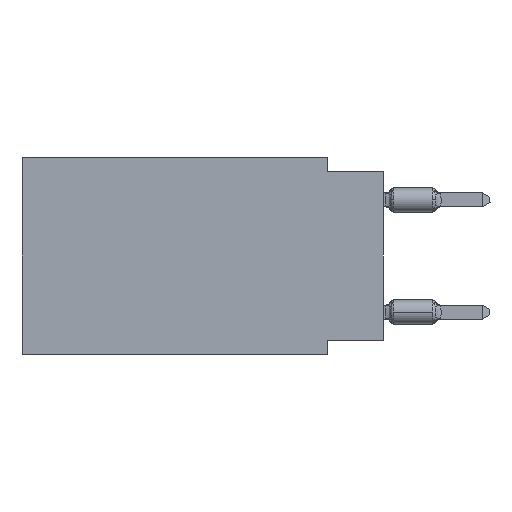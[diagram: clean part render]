
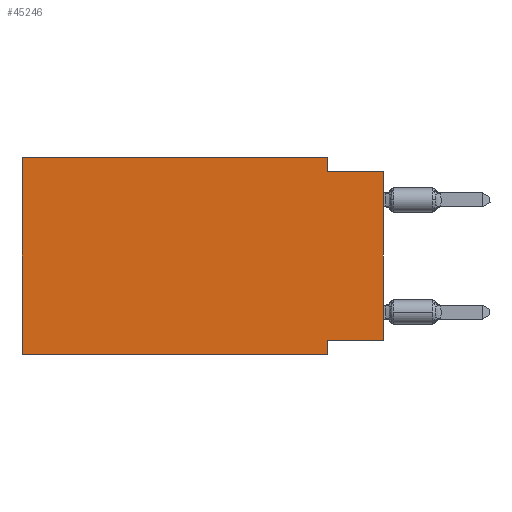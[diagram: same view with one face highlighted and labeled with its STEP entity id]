
A CAD part, left-side view. The second image highlights one B-rep face of the part: STEP entity #45246.
In plain terms, the highlighted planar face has unit normal (-1, 0, 0).
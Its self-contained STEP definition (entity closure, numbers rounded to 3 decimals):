
#296 = EDGE_CURVE ( 'NONE', #33533, #3834, #25748, .T. ) ;
#450 = EDGE_CURVE ( 'NONE', #44304, #37384, #37799, .T. ) ;
#737 = EDGE_CURVE ( 'NONE', #44304, #5291, #46768, .T. ) ;
#1837 = EDGE_CURVE ( 'NONE', #16240, #5291, #23074, .T. ) ;
#2381 = DIRECTION ( 'NONE',  ( 0., 0., -1. ) ) ;
#3282 = CARTESIAN_POINT ( 'NONE',  ( 0., 16.383, 0. ) ) ;
#3382 = ORIENTED_EDGE ( 'NONE', *, *, #44278, .F. ) ;
#3824 = VECTOR ( 'NONE', #22613, 1000. ) ;
#3834 = VERTEX_POINT ( 'NONE', #31379 ) ;
#3975 = VECTOR ( 'NONE', #30225, 1000. ) ;
#4133 = VECTOR ( 'NONE', #21759, 1000. ) ;
#5291 = VERTEX_POINT ( 'NONE', #43436 ) ;
#5717 = DIRECTION ( 'NONE',  ( 0., -1., 0. ) ) ;
#6751 = DIRECTION ( 'NONE',  ( 0., 0., 1. ) ) ;
#7784 = CARTESIAN_POINT ( 'NONE',  ( 0., 2.54, -8.89 ) ) ;
#7787 = LINE ( 'NONE', #40674, #4133 ) ;
#8104 = VECTOR ( 'NONE', #2381, 1000. ) ;
#8425 = CARTESIAN_POINT ( 'NONE',  ( 0., 2.54, -8.255 ) ) ;
#8451 = CARTESIAN_POINT ( 'NONE',  ( 0., 0., -8.255 ) ) ;
#9737 = CARTESIAN_POINT ( 'NONE',  ( 0., 16.383, -8.89 ) ) ;
#12250 = ORIENTED_EDGE ( 'NONE', *, *, #1837, .F. ) ;
#13616 = ORIENTED_EDGE ( 'NONE', *, *, #34430, .F. ) ;
#13820 = VERTEX_POINT ( 'NONE', #31703 ) ;
#13891 = VERTEX_POINT ( 'NONE', #7784 ) ;
#16240 = VERTEX_POINT ( 'NONE', #46066 ) ;
#16364 = DIRECTION ( 'NONE',  ( 0., 0., -1. ) ) ;
#16374 = LINE ( 'NONE', #30789, #8104 ) ;
#18143 = CARTESIAN_POINT ( 'NONE',  ( 0., 0., 0. ) ) ;
#20020 = AXIS2_PLACEMENT_3D ( 'NONE', #34347, #20596, #16364 ) ;
#20144 = PLANE ( 'NONE',  #20020 ) ;
#20194 = EDGE_CURVE ( 'NONE', #13820, #13891, #20393, .T. ) ;
#20393 = LINE ( 'NONE', #9737, #27009 ) ;
#20596 = DIRECTION ( 'NONE',  ( 1., 0., 0. ) ) ;
#21759 = DIRECTION ( 'NONE',  ( 0., 0., 1. ) ) ;
#22613 = DIRECTION ( 'NONE',  ( 0., 0., -1. ) ) ;
#23074 = LINE ( 'NONE', #37014, #36950 ) ;
#23331 = ORIENTED_EDGE ( 'NONE', *, *, #737, .T. ) ;
#23348 = EDGE_LOOP ( 'NONE', ( #23331, #12250, #3382, #39738, #46183, #35556, #13616, #42332 ) ) ;
#25052 = DIRECTION ( 'NONE',  ( 0., -1., 0. ) ) ;
#25748 = LINE ( 'NONE', #3282, #34151 ) ;
#26410 = CARTESIAN_POINT ( 'NONE',  ( 0., 16.383, 0. ) ) ;
#27009 = VECTOR ( 'NONE', #5717, 1000. ) ;
#29237 = DIRECTION ( 'NONE',  ( 0., -1., 0. ) ) ;
#30225 = DIRECTION ( 'NONE',  ( 0., 1., 0. ) ) ;
#30789 = CARTESIAN_POINT ( 'NONE',  ( 0., 2.54, -8.89 ) ) ;
#31379 = CARTESIAN_POINT ( 'NONE',  ( 0., 2.54, 0. ) ) ;
#31703 = CARTESIAN_POINT ( 'NONE',  ( 0., 16.383, -8.89 ) ) ;
#31709 = FACE_OUTER_BOUND ( 'NONE', #23348, .T. ) ;
#33533 = VERTEX_POINT ( 'NONE', #26410 ) ;
#34151 = VECTOR ( 'NONE', #25052, 1000. ) ;
#34347 = CARTESIAN_POINT ( 'NONE',  ( 0., 16.383, 0. ) ) ;
#34430 = EDGE_CURVE ( 'NONE', #37384, #13891, #16374, .T. ) ;
#35556 = ORIENTED_EDGE ( 'NONE', *, *, #20194, .T. ) ;
#35703 = VECTOR ( 'NONE', #6751, 1000. ) ;
#35761 = EDGE_CURVE ( 'NONE', #13820, #33533, #7787, .T. ) ;
#36950 = VECTOR ( 'NONE', #29237, 1000. ) ;
#37014 = CARTESIAN_POINT ( 'NONE',  ( 0., 0., -0.635 ) ) ;
#37292 = CARTESIAN_POINT ( 'NONE',  ( 0., 2.54, 0. ) ) ;
#37384 = VERTEX_POINT ( 'NONE', #8425 ) ;
#37799 = LINE ( 'NONE', #8451, #3975 ) ;
#39738 = ORIENTED_EDGE ( 'NONE', *, *, #296, .F. ) ;
#40674 = CARTESIAN_POINT ( 'NONE',  ( 0., 16.383, 0. ) ) ;
#42022 = CARTESIAN_POINT ( 'NONE',  ( 0., 0., -8.255 ) ) ;
#42332 = ORIENTED_EDGE ( 'NONE', *, *, #450, .F. ) ;
#43436 = CARTESIAN_POINT ( 'NONE',  ( 0., 0., -0.635 ) ) ;
#44278 = EDGE_CURVE ( 'NONE', #3834, #16240, #44860, .T. ) ;
#44304 = VERTEX_POINT ( 'NONE', #42022 ) ;
#44860 = LINE ( 'NONE', #37292, #3824 ) ;
#45246 = ADVANCED_FACE ( 'NONE', ( #31709 ), #20144, .F. ) ;
#46066 = CARTESIAN_POINT ( 'NONE',  ( 0., 2.54, -0.635 ) ) ;
#46183 = ORIENTED_EDGE ( 'NONE', *, *, #35761, .F. ) ;
#46768 = LINE ( 'NONE', #18143, #35703 ) ;
